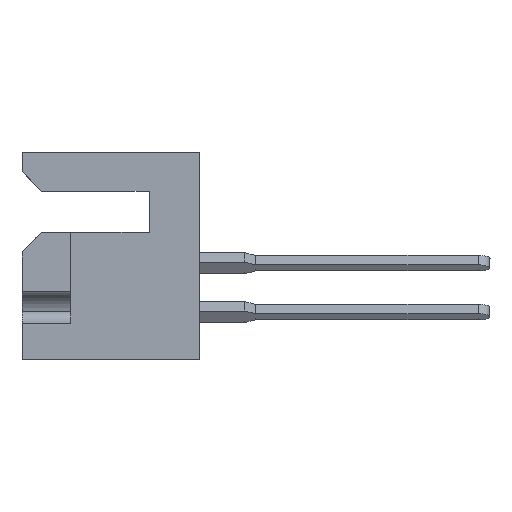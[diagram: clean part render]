
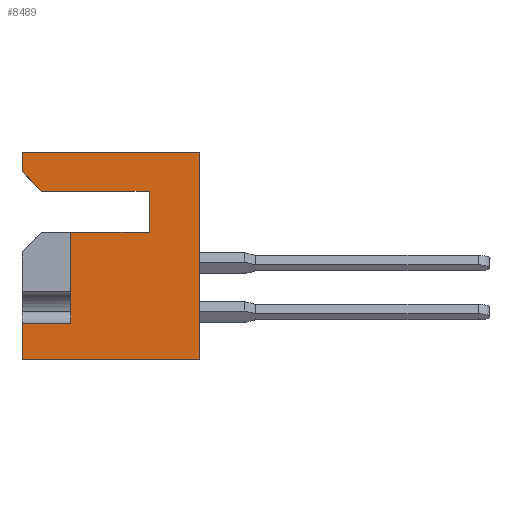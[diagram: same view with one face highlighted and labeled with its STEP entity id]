
A CAD part, left-side view. The second image highlights one B-rep face of the part: STEP entity #8489.
In plain terms, the highlighted planar face has unit normal (-1, 0, 0).
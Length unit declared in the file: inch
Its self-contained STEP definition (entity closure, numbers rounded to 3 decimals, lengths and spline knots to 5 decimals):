
#66 = DIRECTION ( 'NONE',  ( 0., 1., 0. ) ) ;
#370 = VECTOR ( 'NONE', #26469, 39.37008 ) ;
#470 = FACE_OUTER_BOUND ( 'NONE', #26053, .T. ) ;
#559 = CARTESIAN_POINT ( 'NONE',  ( 0., 0.453, -0.531 ) ) ;
#657 = VERTEX_POINT ( 'NONE', #24784 ) ;
#959 = CARTESIAN_POINT ( 'NONE',  ( 0., 0., 0. ) ) ;
#3093 = ORIENTED_EDGE ( 'NONE', *, *, #3894, .T. ) ;
#3115 = VERTEX_POINT ( 'NONE', #26756 ) ;
#3214 = DIRECTION ( 'NONE',  ( 0., 1., 0. ) ) ;
#3447 = ORIENTED_EDGE ( 'NONE', *, *, #20898, .T. ) ;
#3506 = CARTESIAN_POINT ( 'NONE',  ( 0., 0.403, -0.1 ) ) ;
#3587 = CARTESIAN_POINT ( 'NONE',  ( 0., 0.453, 0. ) ) ;
#3837 = CARTESIAN_POINT ( 'NONE',  ( 0., 0., 0. ) ) ;
#3860 = CARTESIAN_POINT ( 'NONE',  ( 0., 0.128, -0.1 ) ) ;
#3894 = EDGE_CURVE ( 'NONE', #12463, #657, #27007, .T. ) ;
#3991 = CARTESIAN_POINT ( 'NONE',  ( 0., 0.128, -0.205 ) ) ;
#4091 = VERTEX_POINT ( 'NONE', #9084 ) ;
#4347 = DIRECTION ( 'NONE',  ( 0., 0., 1. ) ) ;
#6669 = VECTOR ( 'NONE', #16047, 39.37008 ) ;
#6798 = VERTEX_POINT ( 'NONE', #11505 ) ;
#6943 = CARTESIAN_POINT ( 'NONE',  ( 0., 0.453, -0.05 ) ) ;
#7050 = CARTESIAN_POINT ( 'NONE',  ( 0., 0.453, 0. ) ) ;
#7254 = DIRECTION ( 'NONE',  ( 0., 0., 1. ) ) ;
#7269 = EDGE_CURVE ( 'NONE', #28744, #25402, #14673, .T. ) ;
#7316 = VECTOR ( 'NONE', #3214, 39.37008 ) ;
#7545 = DIRECTION ( 'NONE',  ( 0., 0., 1. ) ) ;
#7642 = CARTESIAN_POINT ( 'NONE',  ( 0., 0.453, 0. ) ) ;
#7852 = VERTEX_POINT ( 'NONE', #3837 ) ;
#8489 = ADVANCED_FACE ( 'NONE', ( #470 ), #27494, .F. ) ;
#8828 = ORIENTED_EDGE ( 'NONE', *, *, #19454, .F. ) ;
#8876 = AXIS2_PLACEMENT_3D ( 'NONE', #3587, #15541, #30086 ) ;
#9084 = CARTESIAN_POINT ( 'NONE',  ( 0., 0.128, -0.205 ) ) ;
#9362 = CARTESIAN_POINT ( 'NONE',  ( 0., 0.453, 0. ) ) ;
#10318 = ORIENTED_EDGE ( 'NONE', *, *, #21808, .T. ) ;
#10599 = DIRECTION ( 'NONE',  ( 0., 0., 1. ) ) ;
#10739 = DIRECTION ( 'NONE',  ( 0., -0.707, -0.707 ) ) ;
#11034 = LINE ( 'NONE', #7050, #18501 ) ;
#11505 = CARTESIAN_POINT ( 'NONE',  ( 0., 0.453, 0. ) ) ;
#12414 = VECTOR ( 'NONE', #10739, 39.37008 ) ;
#12444 = EDGE_CURVE ( 'NONE', #4091, #17227, #24010, .T. ) ;
#12463 = VERTEX_POINT ( 'NONE', #6943 ) ;
#14088 = LINE ( 'NONE', #3991, #6669 ) ;
#14120 = LINE ( 'NONE', #959, #18589 ) ;
#14210 = EDGE_CURVE ( 'NONE', #12463, #6798, #29537, .T. ) ;
#14673 = LINE ( 'NONE', #559, #19514 ) ;
#15541 = DIRECTION ( 'NONE',  ( 1., 0., 0. ) ) ;
#15987 = CARTESIAN_POINT ( 'NONE',  ( 0., 0.328, -0.437 ) ) ;
#16047 = DIRECTION ( 'NONE',  ( 0., 1., 0. ) ) ;
#16464 = EDGE_CURVE ( 'NONE', #4091, #28591, #14088, .T. ) ;
#16829 = DIRECTION ( 'NONE',  ( 0., 0., 1. ) ) ;
#17054 = ORIENTED_EDGE ( 'NONE', *, *, #12444, .F. ) ;
#17143 = CARTESIAN_POINT ( 'NONE',  ( 0., 0., -0.531 ) ) ;
#17227 = VERTEX_POINT ( 'NONE', #3860 ) ;
#17452 = CARTESIAN_POINT ( 'NONE',  ( 0., 0.128, -0.1 ) ) ;
#17814 = VECTOR ( 'NONE', #7545, 39.37008 ) ;
#18242 = LINE ( 'NONE', #7642, #370 ) ;
#18501 = VECTOR ( 'NONE', #7254, 39.37008 ) ;
#18589 = VECTOR ( 'NONE', #10599, 39.37008 ) ;
#18676 = CARTESIAN_POINT ( 'NONE',  ( 0., 0.128, -0.1 ) ) ;
#18709 = VECTOR ( 'NONE', #16829, 39.37008 ) ;
#18868 = ORIENTED_EDGE ( 'NONE', *, *, #21952, .F. ) ;
#19279 = LINE ( 'NONE', #28843, #17814 ) ;
#19454 = EDGE_CURVE ( 'NONE', #17227, #657, #21078, .T. ) ;
#19514 = VECTOR ( 'NONE', #26552, 39.37008 ) ;
#19626 = LINE ( 'NONE', #28364, #24848 ) ;
#19987 = EDGE_CURVE ( 'NONE', #6798, #7852, #18242, .T. ) ;
#20263 = VECTOR ( 'NONE', #4347, 39.37008 ) ;
#20898 = EDGE_CURVE ( 'NONE', #25402, #7852, #14120, .T. ) ;
#21078 = LINE ( 'NONE', #17452, #7316 ) ;
#21684 = VERTEX_POINT ( 'NONE', #15987 ) ;
#21808 = EDGE_CURVE ( 'NONE', #21684, #3115, #19626, .T. ) ;
#21952 = EDGE_CURVE ( 'NONE', #28744, #3115, #11034, .T. ) ;
#22775 = ORIENTED_EDGE ( 'NONE', *, *, #7269, .T. ) ;
#24010 = LINE ( 'NONE', #18676, #20263 ) ;
#24339 = ORIENTED_EDGE ( 'NONE', *, *, #26019, .F. ) ;
#24784 = CARTESIAN_POINT ( 'NONE',  ( 0., 0.403, -0.1 ) ) ;
#24848 = VECTOR ( 'NONE', #66, 39.37008 ) ;
#25402 = VERTEX_POINT ( 'NONE', #17143 ) ;
#25751 = ORIENTED_EDGE ( 'NONE', *, *, #16464, .T. ) ;
#26019 = EDGE_CURVE ( 'NONE', #21684, #28591, #19279, .T. ) ;
#26053 = EDGE_LOOP ( 'NONE', ( #10318, #18868, #22775, #3447, #26213, #26720, #3093, #8828, #17054, #25751, #24339 ) ) ;
#26213 = ORIENTED_EDGE ( 'NONE', *, *, #19987, .F. ) ;
#26469 = DIRECTION ( 'NONE',  ( 0., -1., 0. ) ) ;
#26552 = DIRECTION ( 'NONE',  ( 0., -1., 0. ) ) ;
#26720 = ORIENTED_EDGE ( 'NONE', *, *, #14210, .F. ) ;
#26756 = CARTESIAN_POINT ( 'NONE',  ( 0., 0.453, -0.437 ) ) ;
#27007 = LINE ( 'NONE', #3506, #12414 ) ;
#27152 = CARTESIAN_POINT ( 'NONE',  ( 0., 0.328, -0.205 ) ) ;
#27494 = PLANE ( 'NONE',  #8876 ) ;
#28364 = CARTESIAN_POINT ( 'NONE',  ( 0., 0.328, -0.437 ) ) ;
#28591 = VERTEX_POINT ( 'NONE', #27152 ) ;
#28744 = VERTEX_POINT ( 'NONE', #30780 ) ;
#28843 = CARTESIAN_POINT ( 'NONE',  ( 0., 0.328, -0.205 ) ) ;
#29537 = LINE ( 'NONE', #9362, #18709 ) ;
#30086 = DIRECTION ( 'NONE',  ( 0., 0., -1. ) ) ;
#30780 = CARTESIAN_POINT ( 'NONE',  ( 0., 0.453, -0.531 ) ) ;
